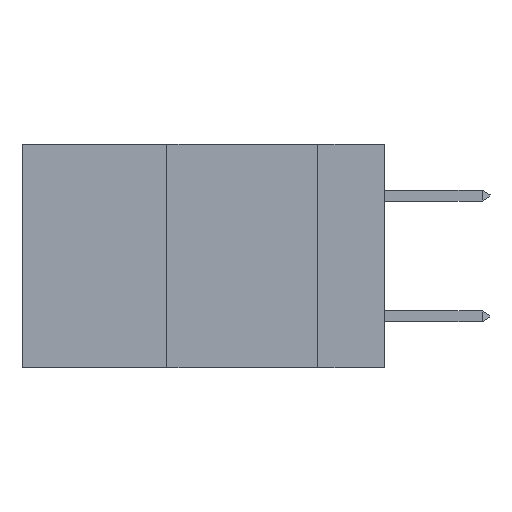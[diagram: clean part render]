
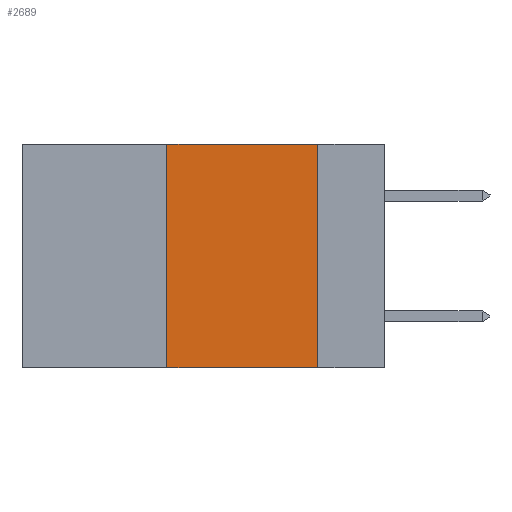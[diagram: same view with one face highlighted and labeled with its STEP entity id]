
A CAD part, left-side view. The second image highlights one B-rep face of the part: STEP entity #2689.
In plain terms, the highlighted planar face has unit normal (-1, 0, 0).
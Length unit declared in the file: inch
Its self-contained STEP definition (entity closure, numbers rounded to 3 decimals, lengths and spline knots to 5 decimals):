
#2470 = CARTESIAN_POINT ( 'NONE',  ( 0., 0.6, 0. ) ) ;
#2499 = EDGE_CURVE ( 'NONE', #20885, #18963, #4315, .T. ) ;
#2689 = ADVANCED_FACE ( 'NONE', ( #23360 ), #21867, .F. ) ;
#2716 = LINE ( 'NONE', #2470, #6173 ) ;
#2831 = VERTEX_POINT ( 'NONE', #5661 ) ;
#3164 = CARTESIAN_POINT ( 'NONE',  ( 0., 0.36, 0. ) ) ;
#4105 = ORIENTED_EDGE ( 'NONE', *, *, #25974, .F. ) ;
#4208 = DIRECTION ( 'NONE',  ( 1., 0., 0. ) ) ;
#4315 = LINE ( 'NONE', #3164, #6403 ) ;
#4951 = CARTESIAN_POINT ( 'NONE',  ( 0., 0.36, 0. ) ) ;
#5661 = CARTESIAN_POINT ( 'NONE',  ( 0., 0.11, 0. ) ) ;
#6173 = VECTOR ( 'NONE', #15492, 39.37008 ) ;
#6403 = VECTOR ( 'NONE', #20901, 39.37008 ) ;
#8951 = CARTESIAN_POINT ( 'NONE',  ( 0., 0.6, -0.37 ) ) ;
#10768 = ORIENTED_EDGE ( 'NONE', *, *, #12503, .T. ) ;
#10786 = DIRECTION ( 'NONE',  ( 0., -1., 0. ) ) ;
#11250 = VECTOR ( 'NONE', #10786, 39.37008 ) ;
#11620 = CARTESIAN_POINT ( 'NONE',  ( 0., 0.36, -0.37 ) ) ;
#11999 = VERTEX_POINT ( 'NONE', #19712 ) ;
#12503 = EDGE_CURVE ( 'NONE', #20885, #11999, #17821, .T. ) ;
#12753 = CARTESIAN_POINT ( 'NONE',  ( 0., 0.11, 0. ) ) ;
#15492 = DIRECTION ( 'NONE',  ( 0., -1., 0. ) ) ;
#15823 = ORIENTED_EDGE ( 'NONE', *, *, #2499, .F. ) ;
#16495 = AXIS2_PLACEMENT_3D ( 'NONE', #17264, #4208, #22273 ) ;
#17264 = CARTESIAN_POINT ( 'NONE',  ( 0., 0.6, 0. ) ) ;
#17821 = LINE ( 'NONE', #8951, #11250 ) ;
#18963 = VERTEX_POINT ( 'NONE', #4951 ) ;
#19215 = DIRECTION ( 'NONE',  ( 0., 0., -1. ) ) ;
#19712 = CARTESIAN_POINT ( 'NONE',  ( 0., 0.11, -0.37 ) ) ;
#19832 = EDGE_LOOP ( 'NONE', ( #4105, #21822, #15823, #10768 ) ) ;
#20885 = VERTEX_POINT ( 'NONE', #11620 ) ;
#20901 = DIRECTION ( 'NONE',  ( 0., 0., 1. ) ) ;
#21822 = ORIENTED_EDGE ( 'NONE', *, *, #27516, .F. ) ;
#21867 = PLANE ( 'NONE',  #16495 ) ;
#22273 = DIRECTION ( 'NONE',  ( 0., 0., -1. ) ) ;
#23360 = FACE_OUTER_BOUND ( 'NONE', #19832, .T. ) ;
#25974 = EDGE_CURVE ( 'NONE', #2831, #11999, #26331, .T. ) ;
#26331 = LINE ( 'NONE', #12753, #27732 ) ;
#27516 = EDGE_CURVE ( 'NONE', #18963, #2831, #2716, .T. ) ;
#27732 = VECTOR ( 'NONE', #19215, 39.37008 ) ;
